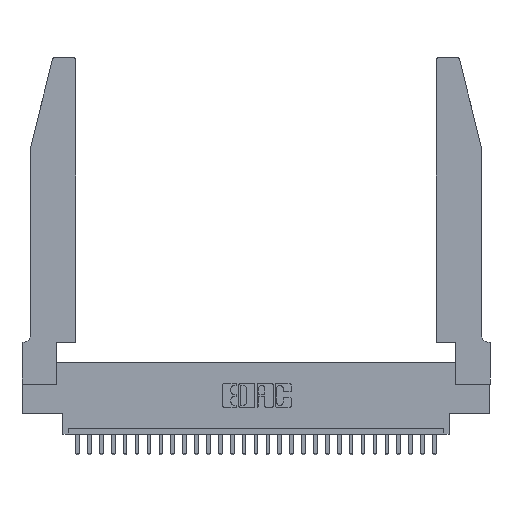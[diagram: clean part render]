
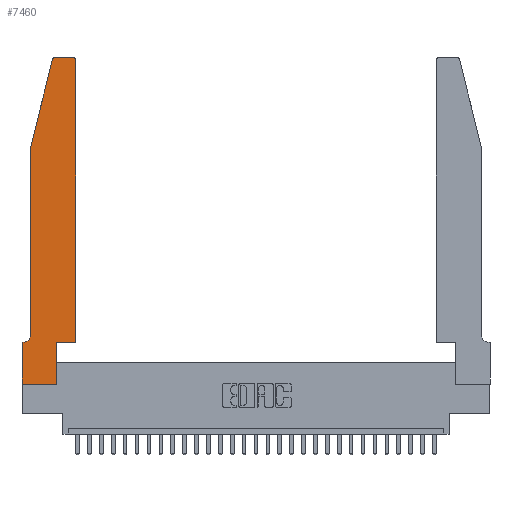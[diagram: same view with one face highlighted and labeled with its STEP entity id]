
A CAD part, top view. The second image highlights one B-rep face of the part: STEP entity #7460.
In plain terms, the highlighted planar face has unit normal (0, 0, 1).
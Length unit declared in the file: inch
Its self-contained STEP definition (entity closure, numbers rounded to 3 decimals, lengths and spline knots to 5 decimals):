
#16 = VERTEX_POINT ( 'NONE', #762 ) ;
#89 = VERTEX_POINT ( 'NONE', #24828 ) ;
#152 = ORIENTED_EDGE ( 'NONE', *, *, #6453, .T. ) ;
#514 = CARTESIAN_POINT ( 'NONE',  ( 0.284, 2.75, 0.37 ) ) ;
#520 = ORIENTED_EDGE ( 'NONE', *, *, #18833, .T. ) ;
#762 = CARTESIAN_POINT ( 'NONE',  ( 0.2865, 0.35, 0.37 ) ) ;
#960 = CARTESIAN_POINT ( 'NONE',  ( 0., 0.35, 0.37 ) ) ;
#1020 = CARTESIAN_POINT ( 'NONE',  ( 0.0755, 2., 0.37 ) ) ;
#1041 = DIRECTION ( 'NONE',  ( 0., 0., 1. ) ) ;
#1070 = EDGE_CURVE ( 'NONE', #11165, #16, #19336, .T. ) ;
#1460 = DIRECTION ( 'NONE',  ( 0., 0., 1. ) ) ;
#1961 = AXIS2_PLACEMENT_3D ( 'NONE', #7247, #1041, #2629 ) ;
#2179 = CARTESIAN_POINT ( 'NONE',  ( 0.4505, 0.35, 0.37 ) ) ;
#2213 = DIRECTION ( 'NONE',  ( 0., 1., 0. ) ) ;
#2402 = VERTEX_POINT ( 'NONE', #7049 ) ;
#2598 = ORIENTED_EDGE ( 'NONE', *, *, #27229, .T. ) ;
#2629 = DIRECTION ( 'NONE',  ( 1., 0., 0. ) ) ;
#3280 = CARTESIAN_POINT ( 'NONE',  ( 0.2865, 0., 0.37 ) ) ;
#3768 = EDGE_CURVE ( 'NONE', #17229, #9142, #24277, .T. ) ;
#4074 = VERTEX_POINT ( 'NONE', #20326 ) ;
#4749 = AXIS2_PLACEMENT_3D ( 'NONE', #19770, #8302, #13021 ) ;
#5436 = VECTOR ( 'NONE', #18291, 39.37008 ) ;
#6453 = EDGE_CURVE ( 'NONE', #4074, #26592, #16512, .T. ) ;
#6529 = ORIENTED_EDGE ( 'NONE', *, *, #27784, .T. ) ;
#6732 = CARTESIAN_POINT ( 'NONE',  ( 0.4505, 0.35, 0.37 ) ) ;
#6786 = ORIENTED_EDGE ( 'NONE', *, *, #19809, .T. ) ;
#7049 = CARTESIAN_POINT ( 'NONE',  ( 0.0755, 2., 0.37 ) ) ;
#7247 = CARTESIAN_POINT ( 'NONE',  ( 0.284, 2.72, 0.37 ) ) ;
#7460 = ADVANCED_FACE ( 'NONE', ( #13543 ), #19557, .T. ) ;
#7545 = VECTOR ( 'NONE', #11815, 39.37008 ) ;
#7575 = CARTESIAN_POINT ( 'NONE',  ( 0.2605, 2.75, 0.37 ) ) ;
#7799 = DIRECTION ( 'NONE',  ( 0., 0., 1. ) ) ;
#7855 = DIRECTION ( 'NONE',  ( 0., -1., 0. ) ) ;
#8302 = DIRECTION ( 'NONE',  ( 0., 0., -1. ) ) ;
#8366 = CARTESIAN_POINT ( 'NONE',  ( 0., 0., 0.37 ) ) ;
#8402 = VERTEX_POINT ( 'NONE', #27859 ) ;
#8495 = VECTOR ( 'NONE', #18142, 39.37008 ) ;
#8965 = CARTESIAN_POINT ( 'NONE',  ( 0.2865, 0.35, 0.37 ) ) ;
#9142 = VERTEX_POINT ( 'NONE', #23849 ) ;
#9316 = CARTESIAN_POINT ( 'NONE',  ( 0.0755, 0.42, 0.37 ) ) ;
#9350 = EDGE_CURVE ( 'NONE', #23145, #2402, #24935, .T. ) ;
#9851 = CARTESIAN_POINT ( 'NONE',  ( 0., 0., 0.37 ) ) ;
#10132 = VERTEX_POINT ( 'NONE', #17237 ) ;
#10189 = DIRECTION ( 'NONE',  ( 1., 0., 0. ) ) ;
#10668 = DIRECTION ( 'NONE',  ( 1., 0., 0. ) ) ;
#10875 = VERTEX_POINT ( 'NONE', #28213 ) ;
#11165 = VERTEX_POINT ( 'NONE', #3280 ) ;
#11815 = DIRECTION ( 'NONE',  ( -1., 0., 0. ) ) ;
#12343 = VECTOR ( 'NONE', #28688, 39.37008 ) ;
#13021 = DIRECTION ( 'NONE',  ( -1., 0., 0. ) ) ;
#13035 = CIRCLE ( 'NONE', #29513, 0.03 ) ;
#13543 = FACE_OUTER_BOUND ( 'NONE', #29239, .T. ) ;
#13875 = ORIENTED_EDGE ( 'NONE', *, *, #1070, .T. ) ;
#14373 = ORIENTED_EDGE ( 'NONE', *, *, #24591, .T. ) ;
#15119 = CARTESIAN_POINT ( 'NONE',  ( 0.4205, 2.72, 0.37 ) ) ;
#15896 = CIRCLE ( 'NONE', #1961, 0.03 ) ;
#16214 = CARTESIAN_POINT ( 'NONE',  ( 0.0755, 0.35, 0.37 ) ) ;
#16512 = LINE ( 'NONE', #7575, #22291 ) ;
#16820 = LINE ( 'NONE', #23954, #28362 ) ;
#17229 = VERTEX_POINT ( 'NONE', #9316 ) ;
#17237 = CARTESIAN_POINT ( 'NONE',  ( 0.4505, 2.72, 0.37 ) ) ;
#17838 = LINE ( 'NONE', #2179, #8495 ) ;
#17973 = ORIENTED_EDGE ( 'NONE', *, *, #3768, .T. ) ;
#18142 = DIRECTION ( 'NONE',  ( 0., 1., 0. ) ) ;
#18291 = DIRECTION ( 'NONE',  ( 1., 0., 0. ) ) ;
#18833 = EDGE_CURVE ( 'NONE', #2402, #17229, #16820, .T. ) ;
#19336 = LINE ( 'NONE', #8965, #27277 ) ;
#19557 = PLANE ( 'NONE',  #28907 ) ;
#19621 = DIRECTION ( 'NONE',  ( -1., 0., 0. ) ) ;
#19770 = CARTESIAN_POINT ( 'NONE',  ( 0.0055, 0.42, 0.37 ) ) ;
#19809 = EDGE_CURVE ( 'NONE', #10875, #10132, #17838, .T. ) ;
#20199 = VECTOR ( 'NONE', #10668, 39.37008 ) ;
#20326 = CARTESIAN_POINT ( 'NONE',  ( 0.4205, 2.75, 0.37 ) ) ;
#20416 = CARTESIAN_POINT ( 'NONE',  ( 0.25487, 2.72718, 0.37 ) ) ;
#20576 = EDGE_CURVE ( 'NONE', #89, #8402, #28297, .T. ) ;
#21986 = DIRECTION ( 'NONE',  ( 1., 0., 0. ) ) ;
#22179 = VECTOR ( 'NONE', #25972, 39.37008 ) ;
#22291 = VECTOR ( 'NONE', #19621, 39.37008 ) ;
#23145 = VERTEX_POINT ( 'NONE', #20416 ) ;
#23442 = LINE ( 'NONE', #6732, #5436 ) ;
#23849 = CARTESIAN_POINT ( 'NONE',  ( 0.0055, 0.35, 0.37 ) ) ;
#23954 = CARTESIAN_POINT ( 'NONE',  ( 0.0755, 2., 0.37 ) ) ;
#24277 = CIRCLE ( 'NONE', #4749, 0.07 ) ;
#24481 = LINE ( 'NONE', #16214, #7545 ) ;
#24591 = EDGE_CURVE ( 'NONE', #9142, #89, #24481, .T. ) ;
#24828 = CARTESIAN_POINT ( 'NONE',  ( 0., 0.35, 0.37 ) ) ;
#24935 = LINE ( 'NONE', #1020, #12343 ) ;
#25972 = DIRECTION ( 'NONE',  ( 0., -1., 0. ) ) ;
#26243 = ORIENTED_EDGE ( 'NONE', *, *, #20576, .T. ) ;
#26592 = VERTEX_POINT ( 'NONE', #514 ) ;
#26767 = ORIENTED_EDGE ( 'NONE', *, *, #9350, .T. ) ;
#26963 = ORIENTED_EDGE ( 'NONE', *, *, #27596, .T. ) ;
#27229 = EDGE_CURVE ( 'NONE', #10132, #4074, #13035, .T. ) ;
#27277 = VECTOR ( 'NONE', #2213, 39.37008 ) ;
#27596 = EDGE_CURVE ( 'NONE', #26592, #23145, #15896, .T. ) ;
#27784 = EDGE_CURVE ( 'NONE', #8402, #11165, #28489, .T. ) ;
#27859 = CARTESIAN_POINT ( 'NONE',  ( 0., 0., 0.37 ) ) ;
#28025 = EDGE_CURVE ( 'NONE', #16, #10875, #23442, .T. ) ;
#28213 = CARTESIAN_POINT ( 'NONE',  ( 0.4505, 0.35, 0.37 ) ) ;
#28297 = LINE ( 'NONE', #9851, #22179 ) ;
#28362 = VECTOR ( 'NONE', #7855, 39.37008 ) ;
#28489 = LINE ( 'NONE', #8366, #20199 ) ;
#28688 = DIRECTION ( 'NONE',  ( -0.239, -0.971, 0. ) ) ;
#28907 = AXIS2_PLACEMENT_3D ( 'NONE', #960, #7799, #21986 ) ;
#29239 = EDGE_LOOP ( 'NONE', ( #152, #26963, #26767, #520, #17973, #14373, #26243, #6529, #13875, #29687, #6786, #2598 ) ) ;
#29513 = AXIS2_PLACEMENT_3D ( 'NONE', #15119, #1460, #10189 ) ;
#29687 = ORIENTED_EDGE ( 'NONE', *, *, #28025, .T. ) ;
